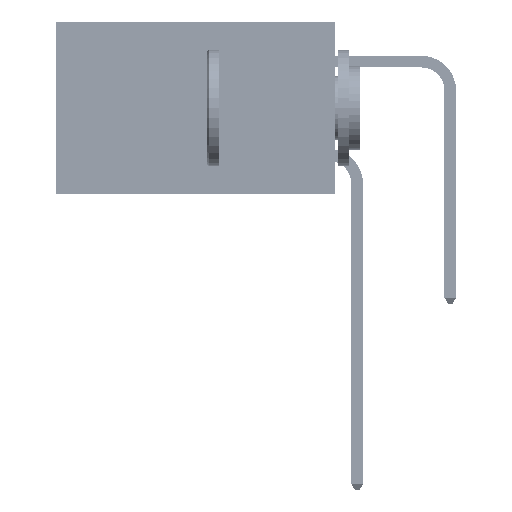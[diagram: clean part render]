
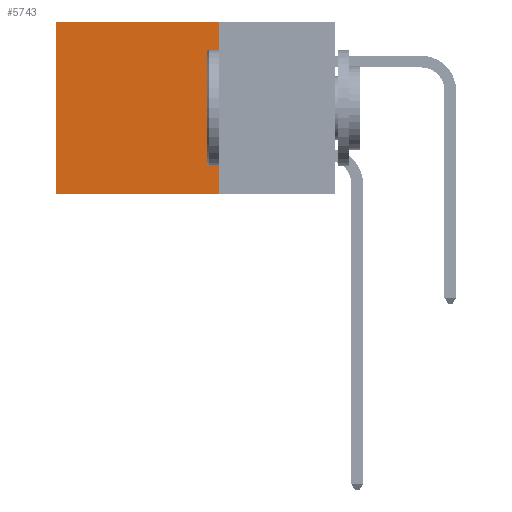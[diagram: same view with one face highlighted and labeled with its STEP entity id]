
A CAD part, left-side view. The second image highlights one B-rep face of the part: STEP entity #5743.
In plain terms, the highlighted planar face has unit normal (-1, 0, 0).
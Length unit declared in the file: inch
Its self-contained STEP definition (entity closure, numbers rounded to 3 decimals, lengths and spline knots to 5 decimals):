
#201 = CARTESIAN_POINT ( 'NONE',  ( 0.2875, 0.25, 0. ) ) ;
#435 = ORIENTED_EDGE ( 'NONE', *, *, #33066, .F. ) ;
#666 = ORIENTED_EDGE ( 'NONE', *, *, #43706, .T. ) ;
#1518 = AXIS2_PLACEMENT_3D ( 'NONE', #14422, #39795, #18055 ) ;
#2579 = VECTOR ( 'NONE', #43516, 39.37008 ) ;
#5743 = ADVANCED_FACE ( 'NONE', ( #13076 ), #36145, .F. ) ;
#7482 = VECTOR ( 'NONE', #15108, 39.37008 ) ;
#7646 = LINE ( 'NONE', #8490, #43946 ) ;
#8490 = CARTESIAN_POINT ( 'NONE',  ( 0.2875, 0.25, 0. ) ) ;
#8811 = ORIENTED_EDGE ( 'NONE', *, *, #22067, .T. ) ;
#9023 = DIRECTION ( 'NONE',  ( 0., 0., -1. ) ) ;
#9099 = VERTEX_POINT ( 'NONE', #22663 ) ;
#12129 = DIRECTION ( 'NONE',  ( 0., 1., 0. ) ) ;
#13076 = FACE_OUTER_BOUND ( 'NONE', #38569, .T. ) ;
#14422 = CARTESIAN_POINT ( 'NONE',  ( 0.2875, 0.25, 0. ) ) ;
#15108 = DIRECTION ( 'NONE',  ( 0., 0., -1. ) ) ;
#17123 = LINE ( 'NONE', #40484, #7482 ) ;
#17484 = LINE ( 'NONE', #34266, #34539 ) ;
#18055 = DIRECTION ( 'NONE',  ( 0., 0., -1. ) ) ;
#21905 = LINE ( 'NONE', #36546, #2579 ) ;
#22067 = EDGE_CURVE ( 'NONE', #28616, #27408, #17484, .T. ) ;
#22663 = CARTESIAN_POINT ( 'NONE',  ( 0.2875, 0.25, -0.37 ) ) ;
#25620 = EDGE_CURVE ( 'NONE', #33065, #9099, #17123, .T. ) ;
#27408 = VERTEX_POINT ( 'NONE', #28755 ) ;
#28616 = VERTEX_POINT ( 'NONE', #46284 ) ;
#28755 = CARTESIAN_POINT ( 'NONE',  ( 0.2875, 0.6, -0.37 ) ) ;
#31066 = ORIENTED_EDGE ( 'NONE', *, *, #25620, .F. ) ;
#33065 = VERTEX_POINT ( 'NONE', #201 ) ;
#33066 = EDGE_CURVE ( 'NONE', #9099, #27408, #21905, .T. ) ;
#34266 = CARTESIAN_POINT ( 'NONE',  ( 0.2875, 0.6, 0. ) ) ;
#34539 = VECTOR ( 'NONE', #9023, 39.37008 ) ;
#36145 = PLANE ( 'NONE',  #1518 ) ;
#36546 = CARTESIAN_POINT ( 'NONE',  ( 0.2875, 0.25, -0.37 ) ) ;
#38569 = EDGE_LOOP ( 'NONE', ( #8811, #435, #31066, #666 ) ) ;
#39795 = DIRECTION ( 'NONE',  ( 1., 0., 0. ) ) ;
#40484 = CARTESIAN_POINT ( 'NONE',  ( 0.2875, 0.25, 0. ) ) ;
#43516 = DIRECTION ( 'NONE',  ( 0., 1., 0. ) ) ;
#43706 = EDGE_CURVE ( 'NONE', #33065, #28616, #7646, .T. ) ;
#43946 = VECTOR ( 'NONE', #12129, 39.37008 ) ;
#46284 = CARTESIAN_POINT ( 'NONE',  ( 0.2875, 0.6, 0. ) ) ;
